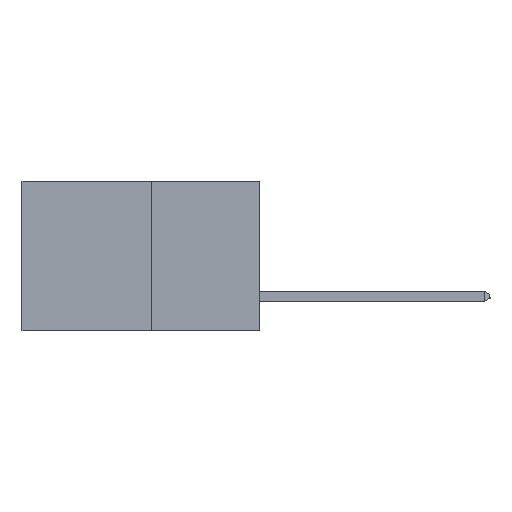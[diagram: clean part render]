
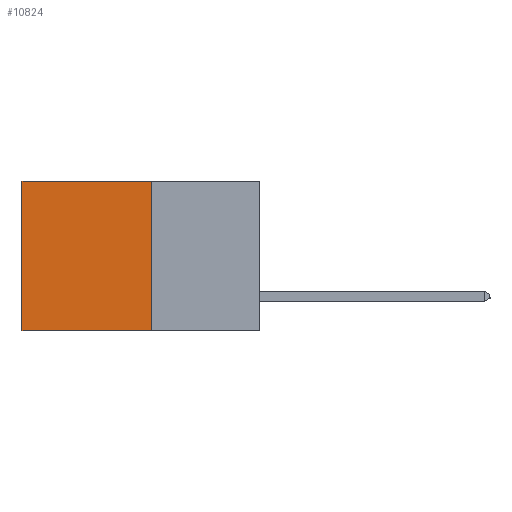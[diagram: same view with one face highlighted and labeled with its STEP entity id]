
A CAD part, left-side view. The second image highlights one B-rep face of the part: STEP entity #10824.
In plain terms, the highlighted planar face has unit normal (-1, 0, 0).
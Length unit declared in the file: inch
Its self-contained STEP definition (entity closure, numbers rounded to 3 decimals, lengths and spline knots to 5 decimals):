
#275 = PLANE ( 'NONE',  #15230 ) ;
#988 = ORIENTED_EDGE ( 'NONE', *, *, #1555, .T. ) ;
#1126 = CARTESIAN_POINT ( 'NONE',  ( 0.277, 0.27, -0.37 ) ) ;
#1207 = VECTOR ( 'NONE', #1903, 39.37008 ) ;
#1555 = EDGE_CURVE ( 'NONE', #11242, #19373, #19248, .T. ) ;
#1903 = DIRECTION ( 'NONE',  ( 0., 1., 0. ) ) ;
#1913 = DIRECTION ( 'NONE',  ( 1., 0., 0. ) ) ;
#3442 = CARTESIAN_POINT ( 'NONE',  ( 0.277, 0.27, -0.37 ) ) ;
#5847 = VECTOR ( 'NONE', #10289, 39.37008 ) ;
#6366 = LINE ( 'NONE', #8664, #5847 ) ;
#6534 = EDGE_CURVE ( 'NONE', #16266, #11242, #13998, .T. ) ;
#6998 = VECTOR ( 'NONE', #13452, 39.37008 ) ;
#7896 = EDGE_CURVE ( 'NONE', #16266, #16566, #11159, .T. ) ;
#8063 = FACE_OUTER_BOUND ( 'NONE', #16992, .T. ) ;
#8664 = CARTESIAN_POINT ( 'NONE',  ( 0.277, 0.27, -0.37 ) ) ;
#9014 = ORIENTED_EDGE ( 'NONE', *, *, #6534, .T. ) ;
#9905 = DIRECTION ( 'NONE',  ( 0., 0., -1. ) ) ;
#10036 = CARTESIAN_POINT ( 'NONE',  ( 0.277, 0.27, 0. ) ) ;
#10289 = DIRECTION ( 'NONE',  ( 0., 1., 0. ) ) ;
#10824 = ADVANCED_FACE ( 'NONE', ( #8063 ), #275, .F. ) ;
#11159 = LINE ( 'NONE', #11438, #19167 ) ;
#11242 = VERTEX_POINT ( 'NONE', #17295 ) ;
#11438 = CARTESIAN_POINT ( 'NONE',  ( 0.277, 0.27, -0.37 ) ) ;
#12400 = CARTESIAN_POINT ( 'NONE',  ( 0.277, 0.59, -0.37 ) ) ;
#12477 = CARTESIAN_POINT ( 'NONE',  ( 0.277, 0.59, -0.37 ) ) ;
#13123 = DIRECTION ( 'NONE',  ( 0., 0., -1. ) ) ;
#13452 = DIRECTION ( 'NONE',  ( 0., 0., -1. ) ) ;
#13579 = ORIENTED_EDGE ( 'NONE', *, *, #17054, .F. ) ;
#13998 = LINE ( 'NONE', #14717, #1207 ) ;
#14493 = ORIENTED_EDGE ( 'NONE', *, *, #7896, .F. ) ;
#14717 = CARTESIAN_POINT ( 'NONE',  ( 0.277, 0.27, 0. ) ) ;
#15230 = AXIS2_PLACEMENT_3D ( 'NONE', #3442, #1913, #13123 ) ;
#16266 = VERTEX_POINT ( 'NONE', #10036 ) ;
#16566 = VERTEX_POINT ( 'NONE', #1126 ) ;
#16992 = EDGE_LOOP ( 'NONE', ( #988, #13579, #14493, #9014 ) ) ;
#17054 = EDGE_CURVE ( 'NONE', #16566, #19373, #6366, .T. ) ;
#17295 = CARTESIAN_POINT ( 'NONE',  ( 0.277, 0.59, 0. ) ) ;
#19167 = VECTOR ( 'NONE', #9905, 39.37008 ) ;
#19248 = LINE ( 'NONE', #12477, #6998 ) ;
#19373 = VERTEX_POINT ( 'NONE', #12400 ) ;
